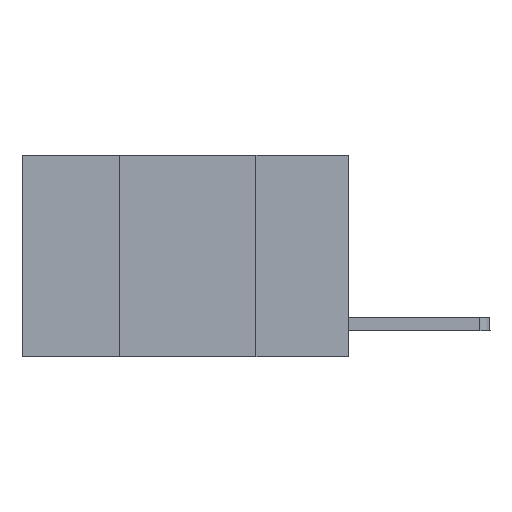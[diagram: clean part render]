
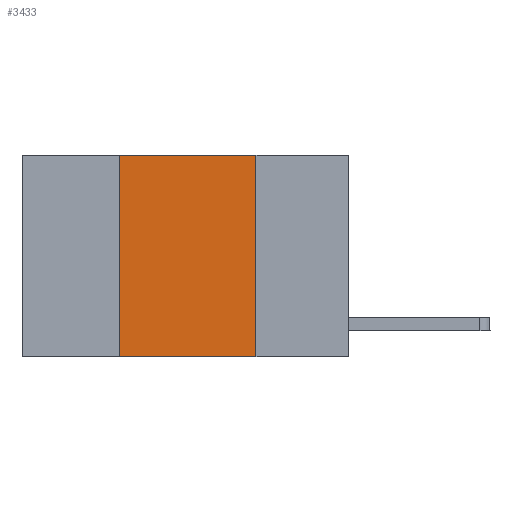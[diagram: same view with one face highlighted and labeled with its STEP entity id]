
A CAD part, left-side view. The second image highlights one B-rep face of the part: STEP entity #3433.
In plain terms, the highlighted planar face has unit normal (-1, 0, 0).
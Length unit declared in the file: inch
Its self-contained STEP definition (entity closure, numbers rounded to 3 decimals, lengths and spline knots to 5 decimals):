
#143 = FACE_OUTER_BOUND ( 'NONE', #8926, .T. ) ;
#225 = VERTEX_POINT ( 'NONE', #3355 ) ;
#399 = DIRECTION ( 'NONE',  ( 0., 0., 1. ) ) ;
#587 = CARTESIAN_POINT ( 'NONE',  ( 0., 0.17, 0. ) ) ;
#798 = VECTOR ( 'NONE', #5072, 39.37008 ) ;
#974 = VECTOR ( 'NONE', #399, 39.37008 ) ;
#982 = DIRECTION ( 'NONE',  ( 0., 0., -1. ) ) ;
#1486 = LINE ( 'NONE', #7416, #2781 ) ;
#1674 = EDGE_CURVE ( 'NONE', #2889, #225, #1486, .T. ) ;
#2053 = CARTESIAN_POINT ( 'NONE',  ( 0., 0.42, 0. ) ) ;
#2060 = ORIENTED_EDGE ( 'NONE', *, *, #6812, .F. ) ;
#2781 = VECTOR ( 'NONE', #9142, 39.37008 ) ;
#2889 = VERTEX_POINT ( 'NONE', #3769 ) ;
#3288 = LINE ( 'NONE', #6720, #798 ) ;
#3355 = CARTESIAN_POINT ( 'NONE',  ( 0., 0.17, 0. ) ) ;
#3433 = ADVANCED_FACE ( 'NONE', ( #143 ), #7797, .F. ) ;
#3703 = DIRECTION ( 'NONE',  ( 1., 0., 0. ) ) ;
#3769 = CARTESIAN_POINT ( 'NONE',  ( 0., 0.42, 0. ) ) ;
#4133 = DIRECTION ( 'NONE',  ( 0., 0., -1. ) ) ;
#5072 = DIRECTION ( 'NONE',  ( 0., -1., 0. ) ) ;
#5807 = VERTEX_POINT ( 'NONE', #8488 ) ;
#5864 = ORIENTED_EDGE ( 'NONE', *, *, #1674, .F. ) ;
#6017 = VERTEX_POINT ( 'NONE', #9730 ) ;
#6720 = CARTESIAN_POINT ( 'NONE',  ( 0., 0.6, -0.37 ) ) ;
#6812 = EDGE_CURVE ( 'NONE', #225, #5807, #7394, .T. ) ;
#7213 = LINE ( 'NONE', #2053, #974 ) ;
#7394 = LINE ( 'NONE', #587, #9282 ) ;
#7416 = CARTESIAN_POINT ( 'NONE',  ( 0., 0.6, 0. ) ) ;
#7797 = PLANE ( 'NONE',  #10026 ) ;
#8312 = EDGE_CURVE ( 'NONE', #6017, #5807, #3288, .T. ) ;
#8475 = ORIENTED_EDGE ( 'NONE', *, *, #8312, .T. ) ;
#8488 = CARTESIAN_POINT ( 'NONE',  ( 0., 0.17, -0.37 ) ) ;
#8503 = EDGE_CURVE ( 'NONE', #6017, #2889, #7213, .T. ) ;
#8926 = EDGE_LOOP ( 'NONE', ( #2060, #5864, #10638, #8475 ) ) ;
#9142 = DIRECTION ( 'NONE',  ( 0., -1., 0. ) ) ;
#9282 = VECTOR ( 'NONE', #4133, 39.37008 ) ;
#9730 = CARTESIAN_POINT ( 'NONE',  ( 0., 0.42, -0.37 ) ) ;
#10026 = AXIS2_PLACEMENT_3D ( 'NONE', #10352, #3703, #982 ) ;
#10352 = CARTESIAN_POINT ( 'NONE',  ( 0., 0.6, 0. ) ) ;
#10638 = ORIENTED_EDGE ( 'NONE', *, *, #8503, .F. ) ;
